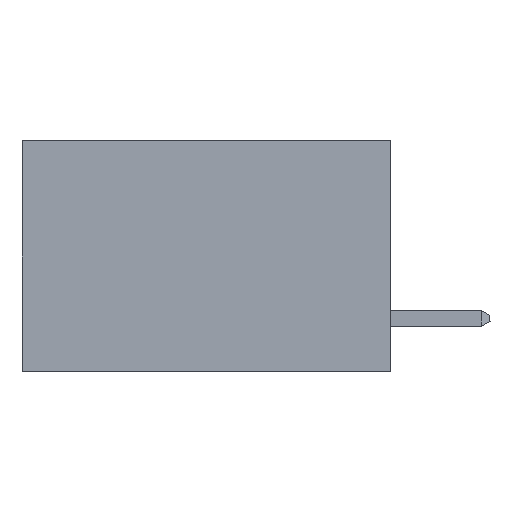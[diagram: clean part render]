
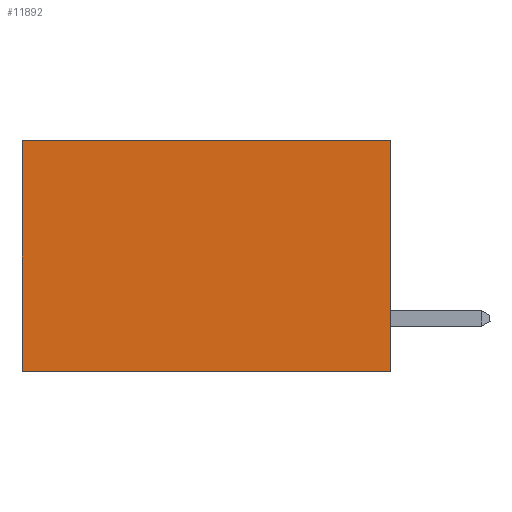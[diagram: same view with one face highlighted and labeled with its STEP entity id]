
A CAD part, left-side view. The second image highlights one B-rep face of the part: STEP entity #11892.
In plain terms, the highlighted planar face has unit normal (-1, 0, 0).
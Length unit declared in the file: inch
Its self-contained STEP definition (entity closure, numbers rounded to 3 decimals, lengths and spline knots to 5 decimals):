
#1196 = LINE ( 'NONE', #29357, #24155 ) ;
#1363 = LINE ( 'NONE', #15415, #25036 ) ;
#1686 = CARTESIAN_POINT ( 'NONE',  ( 0.277, 0., -0.37 ) ) ;
#1696 = CARTESIAN_POINT ( 'NONE',  ( 0.277, 0., -0.37 ) ) ;
#2058 = VERTEX_POINT ( 'NONE', #1696 ) ;
#2774 = CARTESIAN_POINT ( 'NONE',  ( 0.277, 0., 0. ) ) ;
#2832 = EDGE_CURVE ( 'NONE', #15631, #27466, #1196, .T. ) ;
#2980 = DIRECTION ( 'NONE',  ( 0., 1., 0. ) ) ;
#3948 = DIRECTION ( 'NONE',  ( 0., 0., -1. ) ) ;
#6814 = DIRECTION ( 'NONE',  ( 0., 0., -1. ) ) ;
#7476 = CARTESIAN_POINT ( 'NONE',  ( 0.277, 0., 0. ) ) ;
#8008 = FACE_OUTER_BOUND ( 'NONE', #10964, .T. ) ;
#8524 = DIRECTION ( 'NONE',  ( 0., 1., 0. ) ) ;
#8683 = EDGE_CURVE ( 'NONE', #2058, #27466, #20153, .T. ) ;
#9765 = ORIENTED_EDGE ( 'NONE', *, *, #21124, .F. ) ;
#9817 = DIRECTION ( 'NONE',  ( 0., 0., -1. ) ) ;
#10964 = EDGE_LOOP ( 'NONE', ( #28501, #17972, #9765, #12607 ) ) ;
#11077 = CARTESIAN_POINT ( 'NONE',  ( 0.277, 0.59, -0.37 ) ) ;
#11892 = ADVANCED_FACE ( 'NONE', ( #8008 ), #21330, .F. ) ;
#12607 = ORIENTED_EDGE ( 'NONE', *, *, #25884, .T. ) ;
#13327 = VECTOR ( 'NONE', #2980, 39.37008 ) ;
#14372 = CARTESIAN_POINT ( 'NONE',  ( 0.277, 0., -0.37 ) ) ;
#15415 = CARTESIAN_POINT ( 'NONE',  ( 0.277, 0., -0.37 ) ) ;
#15631 = VERTEX_POINT ( 'NONE', #19062 ) ;
#17283 = AXIS2_PLACEMENT_3D ( 'NONE', #14372, #23632, #9817 ) ;
#17972 = ORIENTED_EDGE ( 'NONE', *, *, #8683, .F. ) ;
#18718 = VECTOR ( 'NONE', #8524, 39.37008 ) ;
#18929 = VERTEX_POINT ( 'NONE', #2774 ) ;
#19062 = CARTESIAN_POINT ( 'NONE',  ( 0.277, 0.59, 0. ) ) ;
#19747 = LINE ( 'NONE', #7476, #13327 ) ;
#20153 = LINE ( 'NONE', #1686, #18718 ) ;
#21124 = EDGE_CURVE ( 'NONE', #18929, #2058, #1363, .T. ) ;
#21330 = PLANE ( 'NONE',  #17283 ) ;
#23632 = DIRECTION ( 'NONE',  ( 1., 0., 0. ) ) ;
#24155 = VECTOR ( 'NONE', #6814, 39.37008 ) ;
#25036 = VECTOR ( 'NONE', #3948, 39.37008 ) ;
#25884 = EDGE_CURVE ( 'NONE', #18929, #15631, #19747, .T. ) ;
#27466 = VERTEX_POINT ( 'NONE', #11077 ) ;
#28501 = ORIENTED_EDGE ( 'NONE', *, *, #2832, .T. ) ;
#29357 = CARTESIAN_POINT ( 'NONE',  ( 0.277, 0.59, -0.37 ) ) ;
